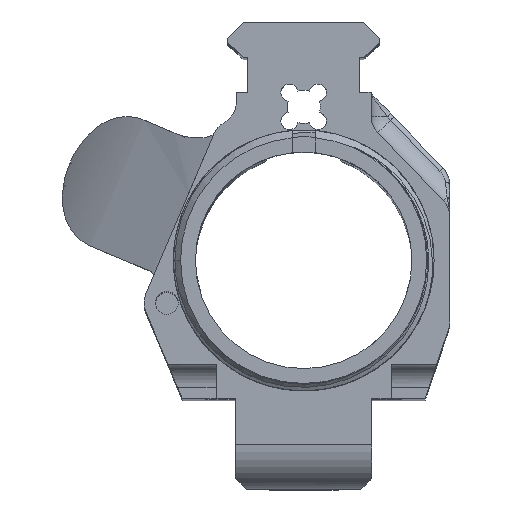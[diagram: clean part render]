
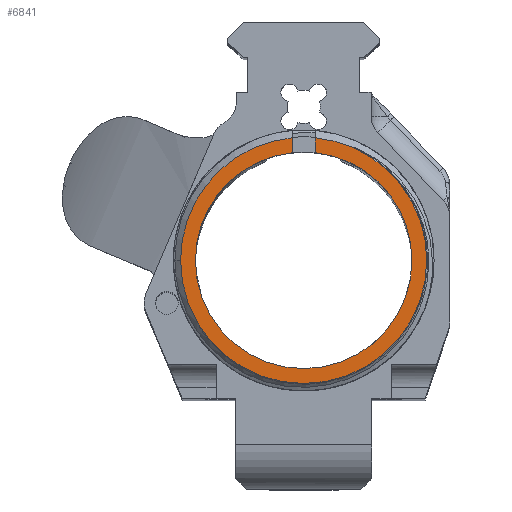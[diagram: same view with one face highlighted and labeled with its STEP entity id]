
A CAD part, top view. The second image highlights one B-rep face of the part: STEP entity #6841.
In plain terms, the highlighted planar face has unit normal (0, 0, 1).
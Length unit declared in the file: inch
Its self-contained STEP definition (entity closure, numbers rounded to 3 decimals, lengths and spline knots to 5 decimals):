
#277 = VERTEX_POINT ( 'NONE', #12828 ) ;
#620 = VECTOR ( 'NONE', #8833, 39.37008 ) ;
#1194 = CARTESIAN_POINT ( 'NONE',  ( -0.063, 1.34715, 0.655 ) ) ;
#1646 = FACE_OUTER_BOUND ( 'NONE', #9578, .T. ) ;
#1751 = VERTEX_POINT ( 'NONE', #4427 ) ;
#2362 = DIRECTION ( 'NONE',  ( 0., 0., 1. ) ) ;
#2381 = CIRCLE ( 'NONE', #9546, 0.5935 ) ;
#2712 = CARTESIAN_POINT ( 'NONE',  ( 0., 0.757, 0.655 ) ) ;
#3413 = CARTESIAN_POINT ( 'NONE',  ( -0.5935, 0.757, 0.655 ) ) ;
#3750 = DIRECTION ( 'NONE',  ( 1., 0., 0. ) ) ;
#4047 = CIRCLE ( 'NONE', #13265, 0.675 ) ;
#4066 = ORIENTED_EDGE ( 'NONE', *, *, #18225, .F. ) ;
#4251 = DIRECTION ( 'NONE',  ( 1., 0., 0. ) ) ;
#4427 = CARTESIAN_POINT ( 'NONE',  ( -0.063, 1.42905, 0.655 ) ) ;
#5765 = CARTESIAN_POINT ( 'NONE',  ( 0.675, 0.757, 0.655 ) ) ;
#6354 = DIRECTION ( 'NONE',  ( 0., 0., 1. ) ) ;
#6738 = CARTESIAN_POINT ( 'NONE',  ( 0., 0.757, 0.655 ) ) ;
#6841 = ADVANCED_FACE ( 'NONE', ( #1646 ), #11301, .T. ) ;
#7066 = EDGE_CURVE ( 'NONE', #18295, #12029, #2381, .T. ) ;
#7178 = ORIENTED_EDGE ( 'NONE', *, *, #17828, .F. ) ;
#7301 = EDGE_CURVE ( 'NONE', #277, #11199, #4047, .T. ) ;
#7955 = EDGE_CURVE ( 'NONE', #11199, #15786, #10193, .T. ) ;
#8256 = EDGE_CURVE ( 'NONE', #11559, #12403, #13495, .T. ) ;
#8504 = ORIENTED_EDGE ( 'NONE', *, *, #18763, .T. ) ;
#8582 = CARTESIAN_POINT ( 'NONE',  ( 0., 0.757, 0.655 ) ) ;
#8783 = ORIENTED_EDGE ( 'NONE', *, *, #8256, .F. ) ;
#8833 = DIRECTION ( 'NONE',  ( 0., 1., 0. ) ) ;
#8867 = DIRECTION ( 'NONE',  ( 0., 0., 1. ) ) ;
#8912 = CARTESIAN_POINT ( 'NONE',  ( 0., 0.757, 0.655 ) ) ;
#9162 = LINE ( 'NONE', #14869, #620 ) ;
#9346 = CIRCLE ( 'NONE', #19393, 0.675 ) ;
#9546 = AXIS2_PLACEMENT_3D ( 'NONE', #8912, #19614, #10437 ) ;
#9578 = EDGE_LOOP ( 'NONE', ( #4066, #8504, #10923, #17834, #19495, #8783, #7178, #19072 ) ) ;
#9944 = AXIS2_PLACEMENT_3D ( 'NONE', #18017, #8867, #19567 ) ;
#10088 = DIRECTION ( 'NONE',  ( 1., 0., 0. ) ) ;
#10193 = CIRCLE ( 'NONE', #19679, 0.675 ) ;
#10437 = DIRECTION ( 'NONE',  ( 1., 0., 0. ) ) ;
#10917 = AXIS2_PLACEMENT_3D ( 'NONE', #6738, #12856, #3750 ) ;
#10923 = ORIENTED_EDGE ( 'NONE', *, *, #7301, .T. ) ;
#11199 = VERTEX_POINT ( 'NONE', #5765 ) ;
#11301 = PLANE ( 'NONE',  #10917 ) ;
#11452 = CARTESIAN_POINT ( 'NONE',  ( 0., 0.757, 0.655 ) ) ;
#11559 = VERTEX_POINT ( 'NONE', #15764 ) ;
#11692 = CARTESIAN_POINT ( 'NONE',  ( -0.063, 1.25, 0.655 ) ) ;
#11981 = CARTESIAN_POINT ( 'NONE',  ( 0.063, 1.34715, 0.655 ) ) ;
#12029 = VERTEX_POINT ( 'NONE', #3413 ) ;
#12280 = AXIS2_PLACEMENT_3D ( 'NONE', #2712, #13352, #4251 ) ;
#12403 = VERTEX_POINT ( 'NONE', #11981 ) ;
#12828 = CARTESIAN_POINT ( 'NONE',  ( -0.675, 0.757, 0.655 ) ) ;
#12856 = DIRECTION ( 'NONE',  ( 0., 0., 1. ) ) ;
#12970 = DIRECTION ( 'NONE',  ( 1., 0., 0. ) ) ;
#13265 = AXIS2_PLACEMENT_3D ( 'NONE', #11452, #2362, #12970 ) ;
#13352 = DIRECTION ( 'NONE',  ( 0., 0., 1. ) ) ;
#13367 = CARTESIAN_POINT ( 'NONE',  ( 0.063, 1.42905, 0.655 ) ) ;
#13495 = CIRCLE ( 'NONE', #9944, 0.5935 ) ;
#13888 = LINE ( 'NONE', #11692, #17528 ) ;
#14777 = DIRECTION ( 'NONE',  ( 0., -1., 0. ) ) ;
#14869 = CARTESIAN_POINT ( 'NONE',  ( 0.063, 1.25, 0.655 ) ) ;
#15468 = CARTESIAN_POINT ( 'NONE',  ( 0., 0.757, 0.655 ) ) ;
#15764 = CARTESIAN_POINT ( 'NONE',  ( 0.5935, 0.757, 0.655 ) ) ;
#15786 = VERTEX_POINT ( 'NONE', #13367 ) ;
#16334 = CIRCLE ( 'NONE', #12280, 0.5935 ) ;
#17007 = DIRECTION ( 'NONE',  ( 1., 0., 0. ) ) ;
#17218 = EDGE_CURVE ( 'NONE', #12403, #15786, #9162, .T. ) ;
#17528 = VECTOR ( 'NONE', #14777, 39.37008 ) ;
#17828 = EDGE_CURVE ( 'NONE', #12029, #11559, #16334, .T. ) ;
#17834 = ORIENTED_EDGE ( 'NONE', *, *, #7955, .T. ) ;
#18017 = CARTESIAN_POINT ( 'NONE',  ( 0., 0.757, 0.655 ) ) ;
#18225 = EDGE_CURVE ( 'NONE', #1751, #18295, #13888, .T. ) ;
#18295 = VERTEX_POINT ( 'NONE', #1194 ) ;
#18763 = EDGE_CURVE ( 'NONE', #1751, #277, #9346, .T. ) ;
#19072 = ORIENTED_EDGE ( 'NONE', *, *, #7066, .F. ) ;
#19273 = DIRECTION ( 'NONE',  ( 0., 0., 1. ) ) ;
#19393 = AXIS2_PLACEMENT_3D ( 'NONE', #8582, #19273, #10088 ) ;
#19495 = ORIENTED_EDGE ( 'NONE', *, *, #17218, .F. ) ;
#19567 = DIRECTION ( 'NONE',  ( 1., 0., 0. ) ) ;
#19614 = DIRECTION ( 'NONE',  ( 0., 0., 1. ) ) ;
#19679 = AXIS2_PLACEMENT_3D ( 'NONE', #15468, #6354, #17007 ) ;
